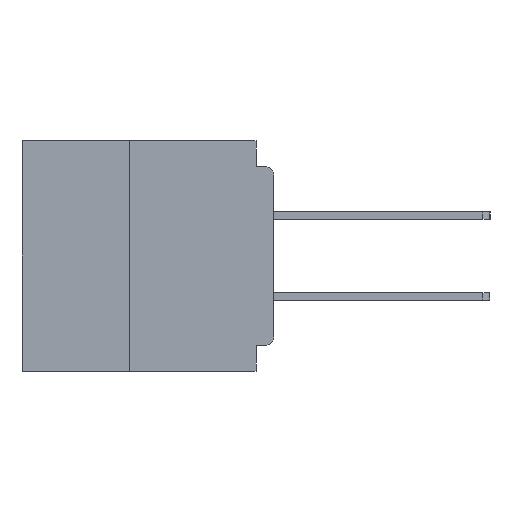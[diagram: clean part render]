
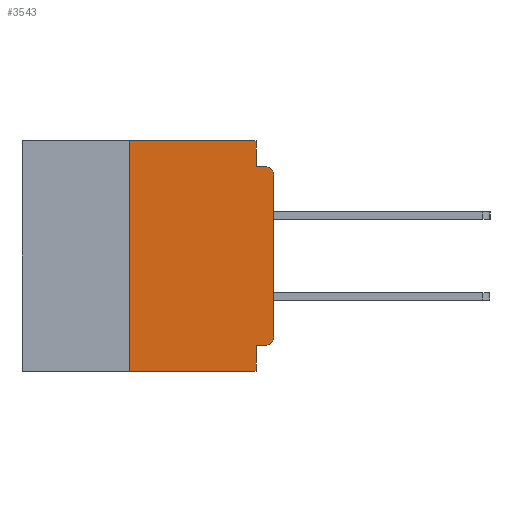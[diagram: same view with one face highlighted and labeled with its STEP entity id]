
A CAD part, left-side view. The second image highlights one B-rep face of the part: STEP entity #3543.
In plain terms, the highlighted planar face has unit normal (-1, 0, 0).
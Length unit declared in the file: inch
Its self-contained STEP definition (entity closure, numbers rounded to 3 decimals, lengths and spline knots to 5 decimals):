
#13 = VERTEX_POINT ( 'NONE', #35754 ) ;
#1370 = LINE ( 'NONE', #35027, #37701 ) ;
#2118 = DIRECTION ( 'NONE',  ( 0., -1., 0. ) ) ;
#3401 = CARTESIAN_POINT ( 'NONE',  ( 0., 0.015, -0.34 ) ) ;
#3543 = ADVANCED_FACE ( 'NONE', ( #39713 ), #29163, .F. ) ;
#4210 = VERTEX_POINT ( 'NONE', #11419 ) ;
#4383 = CARTESIAN_POINT ( 'NONE',  ( 0., 0.437, 0. ) ) ;
#4833 = ORIENTED_EDGE ( 'NONE', *, *, #24068, .F. ) ;
#4972 = VERTEX_POINT ( 'NONE', #24225 ) ;
#5354 = CARTESIAN_POINT ( 'NONE',  ( 0., 0.031, 0. ) ) ;
#5441 = CARTESIAN_POINT ( 'NONE',  ( 0., 0., -0.06 ) ) ;
#5727 = VECTOR ( 'NONE', #19066, 39.37008 ) ;
#5756 = CARTESIAN_POINT ( 'NONE',  ( 0., 0.015, -0.06 ) ) ;
#6709 = DIRECTION ( 'NONE',  ( 0., 0., 1. ) ) ;
#6959 = DIRECTION ( 'NONE',  ( 0., 0., -1. ) ) ;
#7121 = ORIENTED_EDGE ( 'NONE', *, *, #32644, .F. ) ;
#7352 = ORIENTED_EDGE ( 'NONE', *, *, #36266, .T. ) ;
#7652 = LINE ( 'NONE', #12363, #17078 ) ;
#7713 = ORIENTED_EDGE ( 'NONE', *, *, #8429, .T. ) ;
#8429 = EDGE_CURVE ( 'NONE', #22940, #11663, #10920, .T. ) ;
#9061 = CARTESIAN_POINT ( 'NONE',  ( 0., 0., -0.045 ) ) ;
#9103 = LINE ( 'NONE', #34613, #17434 ) ;
#9285 = DIRECTION ( 'NONE',  ( 0., 0., -1. ) ) ;
#9973 = DIRECTION ( 'NONE',  ( 0., 1., 0. ) ) ;
#10920 = CIRCLE ( 'NONE', #16513, 0.015 ) ;
#11412 = CARTESIAN_POINT ( 'NONE',  ( 0., 0., -0.34 ) ) ;
#11419 = CARTESIAN_POINT ( 'NONE',  ( 0., 0.25, 0. ) ) ;
#11538 = VERTEX_POINT ( 'NONE', #31555 ) ;
#11628 = DIRECTION ( 'NONE',  ( 0., 0., -1. ) ) ;
#11663 = VERTEX_POINT ( 'NONE', #11412 ) ;
#11920 = EDGE_CURVE ( 'NONE', #11538, #44548, #23870, .T. ) ;
#12363 = CARTESIAN_POINT ( 'NONE',  ( 0., 0.25, -0.4 ) ) ;
#12515 = VERTEX_POINT ( 'NONE', #12591 ) ;
#12591 = CARTESIAN_POINT ( 'NONE',  ( 0., 0.031, 0. ) ) ;
#14270 = CARTESIAN_POINT ( 'NONE',  ( 0., 0.015, -0.355 ) ) ;
#15362 = VERTEX_POINT ( 'NONE', #5441 ) ;
#15397 = AXIS2_PLACEMENT_3D ( 'NONE', #5756, #30382, #9285 ) ;
#16513 = AXIS2_PLACEMENT_3D ( 'NONE', #3401, #28042, #6959 ) ;
#16895 = ORIENTED_EDGE ( 'NONE', *, *, #35179, .F. ) ;
#17078 = VECTOR ( 'NONE', #36928, 39.37008 ) ;
#17434 = VECTOR ( 'NONE', #45117, 39.37008 ) ;
#17485 = LINE ( 'NONE', #5354, #35038 ) ;
#17542 = DIRECTION ( 'NONE',  ( 0., -1., 0. ) ) ;
#18240 = CARTESIAN_POINT ( 'NONE',  ( 0., 0.031, -0.355 ) ) ;
#19045 = VECTOR ( 'NONE', #9973, 39.37008 ) ;
#19066 = DIRECTION ( 'NONE',  ( 0., -1., 0. ) ) ;
#20507 = CARTESIAN_POINT ( 'NONE',  ( 0., 0., -0.355 ) ) ;
#21052 = EDGE_CURVE ( 'NONE', #11663, #15362, #35802, .T. ) ;
#22170 = ORIENTED_EDGE ( 'NONE', *, *, #39015, .F. ) ;
#22940 = VERTEX_POINT ( 'NONE', #14270 ) ;
#23870 = LINE ( 'NONE', #9061, #30995 ) ;
#24068 = EDGE_CURVE ( 'NONE', #22940, #38271, #38773, .T. ) ;
#24225 = CARTESIAN_POINT ( 'NONE',  ( 0., 0.25, -0.4 ) ) ;
#26458 = VECTOR ( 'NONE', #6709, 39.37008 ) ;
#27185 = ORIENTED_EDGE ( 'NONE', *, *, #21052, .T. ) ;
#28042 = DIRECTION ( 'NONE',  ( -1., 0., 0. ) ) ;
#28091 = CARTESIAN_POINT ( 'NONE',  ( 0., 0.015, -0.045 ) ) ;
#29163 = PLANE ( 'NONE',  #45394 ) ;
#30382 = DIRECTION ( 'NONE',  ( -1., 0., 0. ) ) ;
#30995 = VECTOR ( 'NONE', #2118, 39.37008 ) ;
#31555 = CARTESIAN_POINT ( 'NONE',  ( 0., 0.031, -0.045 ) ) ;
#32644 = EDGE_CURVE ( 'NONE', #4972, #4210, #7652, .T. ) ;
#32698 = DIRECTION ( 'NONE',  ( 1., 0., 0. ) ) ;
#34613 = CARTESIAN_POINT ( 'NONE',  ( 0., 0.031, -0.4 ) ) ;
#35027 = CARTESIAN_POINT ( 'NONE',  ( 0., 0.437, -0.4 ) ) ;
#35038 = VECTOR ( 'NONE', #37036, 39.37008 ) ;
#35179 = EDGE_CURVE ( 'NONE', #38271, #13, #9103, .T. ) ;
#35754 = CARTESIAN_POINT ( 'NONE',  ( 0., 0.031, -0.4 ) ) ;
#35802 = LINE ( 'NONE', #45211, #26458 ) ;
#36105 = EDGE_CURVE ( 'NONE', #4210, #12515, #43075, .T. ) ;
#36266 = EDGE_CURVE ( 'NONE', #15362, #44548, #36525, .T. ) ;
#36525 = CIRCLE ( 'NONE', #15397, 0.015 ) ;
#36894 = ORIENTED_EDGE ( 'NONE', *, *, #36105, .F. ) ;
#36928 = DIRECTION ( 'NONE',  ( 0., 0., 1. ) ) ;
#37036 = DIRECTION ( 'NONE',  ( 0., 0., -1. ) ) ;
#37508 = ORIENTED_EDGE ( 'NONE', *, *, #11920, .F. ) ;
#37701 = VECTOR ( 'NONE', #17542, 39.37008 ) ;
#38271 = VERTEX_POINT ( 'NONE', #18240 ) ;
#38773 = LINE ( 'NONE', #20507, #19045 ) ;
#39015 = EDGE_CURVE ( 'NONE', #12515, #11538, #17485, .T. ) ;
#39713 = FACE_OUTER_BOUND ( 'NONE', #41822, .T. ) ;
#40344 = EDGE_CURVE ( 'NONE', #4972, #13, #1370, .T. ) ;
#41772 = ORIENTED_EDGE ( 'NONE', *, *, #40344, .T. ) ;
#41822 = EDGE_LOOP ( 'NONE', ( #27185, #7352, #37508, #22170, #36894, #7121, #41772, #16895, #4833, #7713 ) ) ;
#43075 = LINE ( 'NONE', #43373, #5727 ) ;
#43373 = CARTESIAN_POINT ( 'NONE',  ( 0., 0.437, 0. ) ) ;
#44548 = VERTEX_POINT ( 'NONE', #28091 ) ;
#45117 = DIRECTION ( 'NONE',  ( 0., 0., -1. ) ) ;
#45211 = CARTESIAN_POINT ( 'NONE',  ( 0., 0., 0. ) ) ;
#45394 = AXIS2_PLACEMENT_3D ( 'NONE', #4383, #32698, #11628 ) ;
